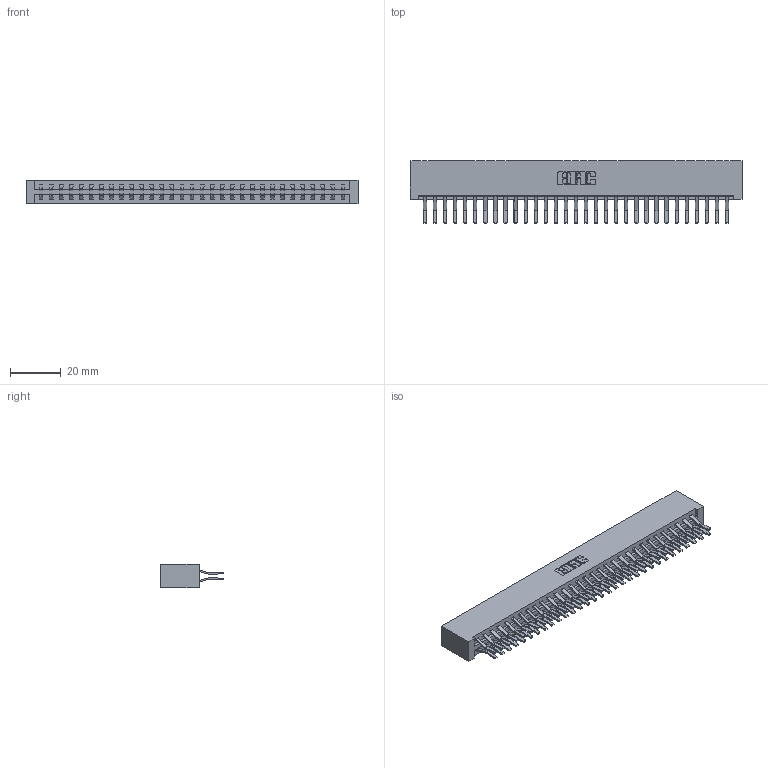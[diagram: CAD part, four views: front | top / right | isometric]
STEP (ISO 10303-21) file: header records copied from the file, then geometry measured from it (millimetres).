
FILE_DESCRIPTION (( 'STEP AP203' ), '1' );
FILE_NAME ('387-062-560-201.STEP', '2019-10-19T15:55:29', ( '' ), ( '' ), 'SwSTEP 2.0', 'SolidWorks 2016', '' );
FILE_SCHEMA (( 'CONFIG_CONTROL_DESIGN' ));
Length unit declared in the file: inch
Products named in the file (3): 337 Part_No Mounting Lugs; 345-292-001_560 Tail; 387-062-560-201
Assembly tree (63 placements, depth 2):
  387-062-560-201
    337 Part_No Mounting Lugs
    345-292-001_560 Tail  x62
Bounding box: 130.71 x 24.78 x 9.4 mm (x, y, z)
Volume: 14795.8 mm3; surface area: 17852.1 mm2
Topology: 63 solids, 63 shells, 3578 faces, 10641 edges, 7010 vertices
Faces by surface type: plane 2422, cylinder 1156
Entity records: 25269 total; most frequent: CARTESIAN_POINT 4266, ORIENTED_EDGE 4202, DIRECTION 3645, EDGE_CURVE 2101, LINE 1977, VECTOR 1977, VERTEX_POINT 1398, AXIS2_PLACEMENT_3D 834
